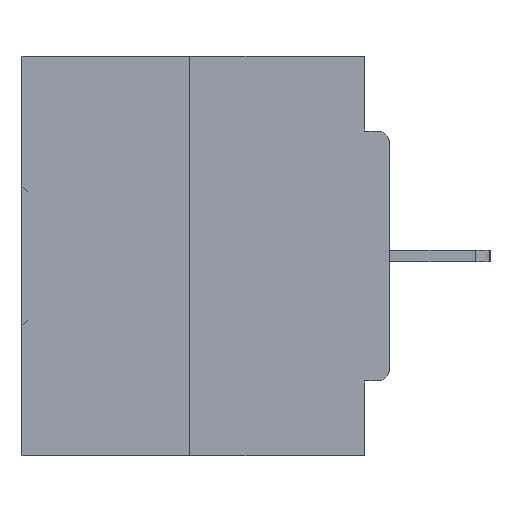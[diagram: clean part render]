
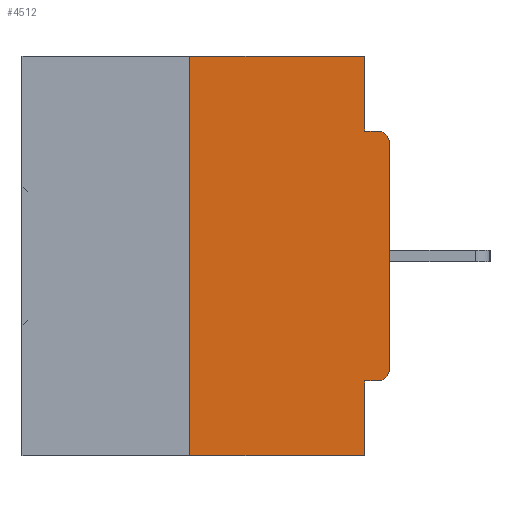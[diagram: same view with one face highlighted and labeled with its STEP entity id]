
A CAD part, left-side view. The second image highlights one B-rep face of the part: STEP entity #4512.
In plain terms, the highlighted planar face has unit normal (-1, 0, 0).
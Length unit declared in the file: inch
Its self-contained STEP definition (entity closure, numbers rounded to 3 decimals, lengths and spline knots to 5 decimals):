
#328 = VERTEX_POINT ( 'NONE', #12897 ) ;
#409 = DIRECTION ( 'NONE',  ( 0., 0., -1. ) ) ;
#519 = DIRECTION ( 'NONE',  ( 0., 0., -1. ) ) ;
#921 = EDGE_CURVE ( 'NONE', #20608, #37975, #26054, .T. ) ;
#1023 = CARTESIAN_POINT ( 'NONE',  ( 0., 0., -0.4065 ) ) ;
#1189 = DIRECTION ( 'NONE',  ( -1., 0., 0. ) ) ;
#1691 = AXIS2_PLACEMENT_3D ( 'NONE', #21971, #1189, #409 ) ;
#1886 = DIRECTION ( 'NONE',  ( 0., 0., 1. ) ) ;
#2834 = EDGE_CURVE ( 'NONE', #328, #11587, #17242, .T. ) ;
#3062 = EDGE_CURVE ( 'NONE', #37975, #4169, #18779, .T. ) ;
#3539 = ORIENTED_EDGE ( 'NONE', *, *, #6157, .F. ) ;
#4169 = VERTEX_POINT ( 'NONE', #32211 ) ;
#4234 = LINE ( 'NONE', #28017, #31198 ) ;
#4478 = PLANE ( 'NONE',  #28005 ) ;
#4512 = ADVANCED_FACE ( 'NONE', ( #34941 ), #4478, .F. ) ;
#6157 = EDGE_CURVE ( 'NONE', #8718, #25644, #8158, .T. ) ;
#7456 = CARTESIAN_POINT ( 'NONE',  ( 0., 0.46, 0. ) ) ;
#8158 = LINE ( 'NONE', #22829, #20726 ) ;
#8718 = VERTEX_POINT ( 'NONE', #13444 ) ;
#10665 = EDGE_CURVE ( 'NONE', #26898, #20608, #25709, .T. ) ;
#10721 = CARTESIAN_POINT ( 'NONE',  ( 0., 0.031, -0.5 ) ) ;
#11587 = VERTEX_POINT ( 'NONE', #13784 ) ;
#11996 = ORIENTED_EDGE ( 'NONE', *, *, #34809, .T. ) ;
#12630 = CARTESIAN_POINT ( 'NONE',  ( 0., 0., -0.3915 ) ) ;
#12897 = CARTESIAN_POINT ( 'NONE',  ( 0., 0.031, -0.4065 ) ) ;
#13164 = EDGE_CURVE ( 'NONE', #25644, #4169, #30683, .T. ) ;
#13444 = CARTESIAN_POINT ( 'NONE',  ( 0., 0.031, 0. ) ) ;
#13710 = CARTESIAN_POINT ( 'NONE',  ( 0., 0.25, 0. ) ) ;
#13784 = CARTESIAN_POINT ( 'NONE',  ( 0., 0.031, -0.5 ) ) ;
#14240 = LINE ( 'NONE', #31711, #35640 ) ;
#14280 = CARTESIAN_POINT ( 'NONE',  ( 0., 0.25, -0.5 ) ) ;
#15357 = EDGE_CURVE ( 'NONE', #15530, #23883, #16508, .T. ) ;
#15530 = VERTEX_POINT ( 'NONE', #14280 ) ;
#15608 = CARTESIAN_POINT ( 'NONE',  ( 0., 0., -0.0935 ) ) ;
#16014 = VECTOR ( 'NONE', #28354, 39.37008 ) ;
#16508 = LINE ( 'NONE', #13710, #31694 ) ;
#17086 = DIRECTION ( 'NONE',  ( 0., 0., 1. ) ) ;
#17242 = LINE ( 'NONE', #10721, #18138 ) ;
#18138 = VECTOR ( 'NONE', #20396, 39.37008 ) ;
#18495 = EDGE_CURVE ( 'NONE', #23883, #8718, #4234, .T. ) ;
#18779 = CIRCLE ( 'NONE', #1691, 0.015 ) ;
#19082 = ORIENTED_EDGE ( 'NONE', *, *, #921, .T. ) ;
#19823 = DIRECTION ( 'NONE',  ( 0., -1., 0. ) ) ;
#19916 = ORIENTED_EDGE ( 'NONE', *, *, #33482, .F. ) ;
#20396 = DIRECTION ( 'NONE',  ( 0., 0., -1. ) ) ;
#20608 = VERTEX_POINT ( 'NONE', #12630 ) ;
#20726 = VECTOR ( 'NONE', #34902, 39.37008 ) ;
#21971 = CARTESIAN_POINT ( 'NONE',  ( 0., 0.015, -0.1085 ) ) ;
#22500 = EDGE_LOOP ( 'NONE', ( #37987, #27535, #11996, #29307, #19916, #30477, #19082, #26918, #23589, #3539 ) ) ;
#22829 = CARTESIAN_POINT ( 'NONE',  ( 0., 0.031, 0. ) ) ;
#23061 = DIRECTION ( 'NONE',  ( 1., 0., 0. ) ) ;
#23589 = ORIENTED_EDGE ( 'NONE', *, *, #13164, .F. ) ;
#23883 = VERTEX_POINT ( 'NONE', #36023 ) ;
#23907 = CARTESIAN_POINT ( 'NONE',  ( 0., 0.015, -0.4065 ) ) ;
#25513 = DIRECTION ( 'NONE',  ( 0., -1., 0. ) ) ;
#25644 = VERTEX_POINT ( 'NONE', #35387 ) ;
#25709 = CIRCLE ( 'NONE', #38933, 0.015 ) ;
#26054 = LINE ( 'NONE', #29043, #34904 ) ;
#26898 = VERTEX_POINT ( 'NONE', #23907 ) ;
#26918 = ORIENTED_EDGE ( 'NONE', *, *, #3062, .T. ) ;
#27535 = ORIENTED_EDGE ( 'NONE', *, *, #15357, .F. ) ;
#27626 = DIRECTION ( 'NONE',  ( -1., 0., 0. ) ) ;
#27741 = LINE ( 'NONE', #1023, #16014 ) ;
#28005 = AXIS2_PLACEMENT_3D ( 'NONE', #7456, #23061, #28652 ) ;
#28017 = CARTESIAN_POINT ( 'NONE',  ( 0., 0.46, 0. ) ) ;
#28354 = DIRECTION ( 'NONE',  ( 0., 1., 0. ) ) ;
#28403 = VECTOR ( 'NONE', #25513, 39.37008 ) ;
#28485 = CARTESIAN_POINT ( 'NONE',  ( 0., 0., -0.1085 ) ) ;
#28652 = DIRECTION ( 'NONE',  ( 0., 0., -1. ) ) ;
#29043 = CARTESIAN_POINT ( 'NONE',  ( 0., 0., 0. ) ) ;
#29307 = ORIENTED_EDGE ( 'NONE', *, *, #2834, .F. ) ;
#30477 = ORIENTED_EDGE ( 'NONE', *, *, #10665, .T. ) ;
#30683 = LINE ( 'NONE', #15608, #28403 ) ;
#30815 = CARTESIAN_POINT ( 'NONE',  ( 0., 0.015, -0.3915 ) ) ;
#31198 = VECTOR ( 'NONE', #36899, 39.37008 ) ;
#31694 = VECTOR ( 'NONE', #17086, 39.37008 ) ;
#31711 = CARTESIAN_POINT ( 'NONE',  ( 0., 0.46, -0.5 ) ) ;
#32211 = CARTESIAN_POINT ( 'NONE',  ( 0., 0.015, -0.0935 ) ) ;
#33482 = EDGE_CURVE ( 'NONE', #26898, #328, #27741, .T. ) ;
#34809 = EDGE_CURVE ( 'NONE', #15530, #11587, #14240, .T. ) ;
#34902 = DIRECTION ( 'NONE',  ( 0., 0., -1. ) ) ;
#34904 = VECTOR ( 'NONE', #1886, 39.37008 ) ;
#34941 = FACE_OUTER_BOUND ( 'NONE', #22500, .T. ) ;
#35387 = CARTESIAN_POINT ( 'NONE',  ( 0., 0.031, -0.0935 ) ) ;
#35640 = VECTOR ( 'NONE', #19823, 39.37008 ) ;
#36023 = CARTESIAN_POINT ( 'NONE',  ( 0., 0.25, 0. ) ) ;
#36899 = DIRECTION ( 'NONE',  ( 0., -1., 0. ) ) ;
#37975 = VERTEX_POINT ( 'NONE', #28485 ) ;
#37987 = ORIENTED_EDGE ( 'NONE', *, *, #18495, .F. ) ;
#38933 = AXIS2_PLACEMENT_3D ( 'NONE', #30815, #27626, #519 ) ;
